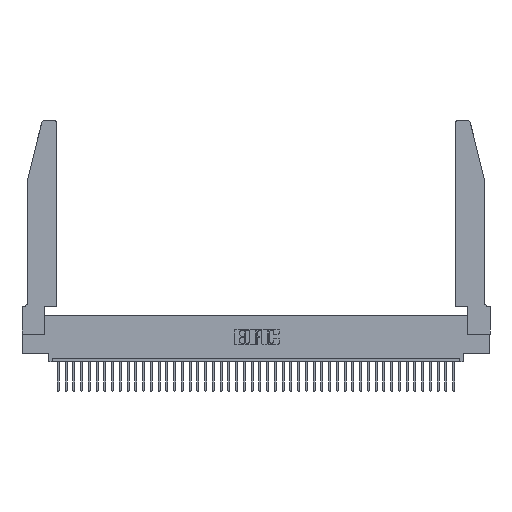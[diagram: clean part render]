
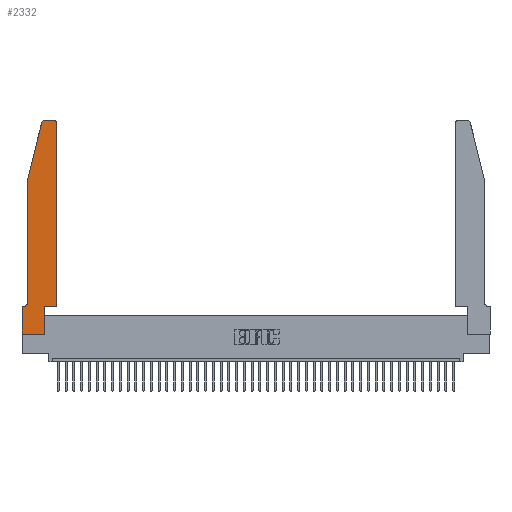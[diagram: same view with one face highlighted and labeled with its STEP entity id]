
A CAD part, top view. The second image highlights one B-rep face of the part: STEP entity #2332.
In plain terms, the highlighted planar face has unit normal (0, 0, 1).
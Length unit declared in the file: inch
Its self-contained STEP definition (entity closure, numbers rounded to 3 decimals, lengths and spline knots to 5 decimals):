
#23 = PLANE ( 'NONE',  #446 ) ;
#157 = DIRECTION ( 'NONE',  ( 1., 0., 0. ) ) ;
#178 = LINE ( 'NONE', #6188, #29043 ) ;
#213 = ORIENTED_EDGE ( 'NONE', *, *, #14156, .T. ) ;
#418 = ORIENTED_EDGE ( 'NONE', *, *, #34478, .T. ) ;
#446 = AXIS2_PLACEMENT_3D ( 'NONE', #26949, #29822, #157 ) ;
#1117 = CARTESIAN_POINT ( 'NONE',  ( 0., 0., 0.37 ) ) ;
#1742 = FACE_OUTER_BOUND ( 'NONE', #40626, .T. ) ;
#1917 = ORIENTED_EDGE ( 'NONE', *, *, #10054, .T. ) ;
#2095 = ORIENTED_EDGE ( 'NONE', *, *, #18398, .T. ) ;
#2332 = ADVANCED_FACE ( 'NONE', ( #1742 ), #23, .T. ) ;
#2423 = DIRECTION ( 'NONE',  ( 0., 1., 0. ) ) ;
#2573 = CARTESIAN_POINT ( 'NONE',  ( 0.2865, 0.35, 0.37 ) ) ;
#3105 = VERTEX_POINT ( 'NONE', #30296 ) ;
#3519 = AXIS2_PLACEMENT_3D ( 'NONE', #18840, #19130, #35691 ) ;
#4041 = EDGE_CURVE ( 'NONE', #3105, #24689, #11425, .T. ) ;
#4183 = CARTESIAN_POINT ( 'NONE',  ( 0.4505, 0.35, 0.37 ) ) ;
#4544 = CARTESIAN_POINT ( 'NONE',  ( 0.4205, 2.72, 0.37 ) ) ;
#4831 = EDGE_CURVE ( 'NONE', #13721, #42676, #30456, .T. ) ;
#4833 = DIRECTION ( 'NONE',  ( 0., 0., 1. ) ) ;
#5234 = CARTESIAN_POINT ( 'NONE',  ( 0.4205, 2.75, 0.37 ) ) ;
#5642 = EDGE_CURVE ( 'NONE', #30776, #18917, #25253, .T. ) ;
#6029 = LINE ( 'NONE', #32280, #40094 ) ;
#6188 = CARTESIAN_POINT ( 'NONE',  ( 0.4505, 0.35, 0.37 ) ) ;
#6521 = DIRECTION ( 'NONE',  ( -1., 0., 0. ) ) ;
#6997 = LINE ( 'NONE', #38324, #8029 ) ;
#7687 = LINE ( 'NONE', #28953, #13379 ) ;
#7872 = CARTESIAN_POINT ( 'NONE',  ( 0.25487, 2.72718, 0.37 ) ) ;
#8029 = VECTOR ( 'NONE', #15065, 39.37008 ) ;
#8715 = LINE ( 'NONE', #2573, #23701 ) ;
#9476 = DIRECTION ( 'NONE',  ( -1., 0., 0. ) ) ;
#9899 = VERTEX_POINT ( 'NONE', #38356 ) ;
#10054 = EDGE_CURVE ( 'NONE', #42676, #26106, #7687, .T. ) ;
#11241 = VECTOR ( 'NONE', #37070, 39.37008 ) ;
#11425 = LINE ( 'NONE', #27756, #39852 ) ;
#11808 = VERTEX_POINT ( 'NONE', #39655 ) ;
#12030 = EDGE_CURVE ( 'NONE', #26106, #30776, #6997, .T. ) ;
#12804 = ORIENTED_EDGE ( 'NONE', *, *, #19382, .T. ) ;
#13379 = VECTOR ( 'NONE', #22488, 39.37008 ) ;
#13721 = VERTEX_POINT ( 'NONE', #31810 ) ;
#14156 = EDGE_CURVE ( 'NONE', #11808, #21584, #38530, .T. ) ;
#14802 = CARTESIAN_POINT ( 'NONE',  ( 0.0755, 0.42, 0.37 ) ) ;
#15065 = DIRECTION ( 'NONE',  ( 0., -1., 0. ) ) ;
#15406 = LINE ( 'NONE', #4183, #11241 ) ;
#16074 = CARTESIAN_POINT ( 'NONE',  ( 0.0055, 0.42, 0.37 ) ) ;
#17065 = ORIENTED_EDGE ( 'NONE', *, *, #4041, .T. ) ;
#18398 = EDGE_CURVE ( 'NONE', #20252, #20653, #8715, .T. ) ;
#18840 = CARTESIAN_POINT ( 'NONE',  ( 0.284, 2.72, 0.37 ) ) ;
#18917 = VERTEX_POINT ( 'NONE', #34940 ) ;
#19130 = DIRECTION ( 'NONE',  ( 0., 0., 1. ) ) ;
#19382 = EDGE_CURVE ( 'NONE', #24689, #20252, #40137, .T. ) ;
#19650 = CARTESIAN_POINT ( 'NONE',  ( 0.2865, 0., 0.37 ) ) ;
#20036 = VECTOR ( 'NONE', #31714, 39.37008 ) ;
#20252 = VERTEX_POINT ( 'NONE', #19650 ) ;
#20653 = VERTEX_POINT ( 'NONE', #28682 ) ;
#20753 = ORIENTED_EDGE ( 'NONE', *, *, #4831, .T. ) ;
#21560 = ORIENTED_EDGE ( 'NONE', *, *, #27192, .T. ) ;
#21584 = VERTEX_POINT ( 'NONE', #5234 ) ;
#22488 = DIRECTION ( 'NONE',  ( -0.239, -0.971, 0. ) ) ;
#22776 = CARTESIAN_POINT ( 'NONE',  ( 0.2605, 2.75, 0.37 ) ) ;
#23701 = VECTOR ( 'NONE', #2423, 39.37008 ) ;
#24460 = EDGE_CURVE ( 'NONE', #20653, #9899, #178, .T. ) ;
#24689 = VERTEX_POINT ( 'NONE', #1117 ) ;
#25253 = CIRCLE ( 'NONE', #33739, 0.07 ) ;
#26106 = VERTEX_POINT ( 'NONE', #31081 ) ;
#26949 = CARTESIAN_POINT ( 'NONE',  ( 0., 0.35, 0.37 ) ) ;
#27192 = EDGE_CURVE ( 'NONE', #9899, #11808, #15406, .T. ) ;
#27292 = LINE ( 'NONE', #22776, #38676 ) ;
#27756 = CARTESIAN_POINT ( 'NONE',  ( 0., 0., 0.37 ) ) ;
#28682 = CARTESIAN_POINT ( 'NONE',  ( 0.2865, 0.35, 0.37 ) ) ;
#28953 = CARTESIAN_POINT ( 'NONE',  ( 0.0755, 2., 0.37 ) ) ;
#29043 = VECTOR ( 'NONE', #39250, 39.37008 ) ;
#29483 = DIRECTION ( 'NONE',  ( 0., 0., -1. ) ) ;
#29822 = DIRECTION ( 'NONE',  ( 0., 0., 1. ) ) ;
#30296 = CARTESIAN_POINT ( 'NONE',  ( 0., 0.35, 0.37 ) ) ;
#30313 = AXIS2_PLACEMENT_3D ( 'NONE', #4544, #4833, #31173 ) ;
#30456 = CIRCLE ( 'NONE', #3519, 0.03 ) ;
#30776 = VERTEX_POINT ( 'NONE', #14802 ) ;
#31048 = DIRECTION ( 'NONE',  ( 0., -1., 0. ) ) ;
#31081 = CARTESIAN_POINT ( 'NONE',  ( 0.0755, 2., 0.37 ) ) ;
#31173 = DIRECTION ( 'NONE',  ( 1., 0., 0. ) ) ;
#31714 = DIRECTION ( 'NONE',  ( 1., 0., 0. ) ) ;
#31810 = CARTESIAN_POINT ( 'NONE',  ( 0.284, 2.75, 0.37 ) ) ;
#32252 = ORIENTED_EDGE ( 'NONE', *, *, #12030, .T. ) ;
#32280 = CARTESIAN_POINT ( 'NONE',  ( 0.0755, 0.35, 0.37 ) ) ;
#33415 = EDGE_CURVE ( 'NONE', #21584, #13721, #27292, .T. ) ;
#33739 = AXIS2_PLACEMENT_3D ( 'NONE', #16074, #29483, #6521 ) ;
#34478 = EDGE_CURVE ( 'NONE', #18917, #3105, #6029, .T. ) ;
#34940 = CARTESIAN_POINT ( 'NONE',  ( 0.0055, 0.35, 0.37 ) ) ;
#35691 = DIRECTION ( 'NONE',  ( 1., 0., 0. ) ) ;
#37070 = DIRECTION ( 'NONE',  ( 0., 1., 0. ) ) ;
#37663 = ORIENTED_EDGE ( 'NONE', *, *, #24460, .T. ) ;
#38324 = CARTESIAN_POINT ( 'NONE',  ( 0.0755, 2., 0.37 ) ) ;
#38356 = CARTESIAN_POINT ( 'NONE',  ( 0.4505, 0.35, 0.37 ) ) ;
#38530 = CIRCLE ( 'NONE', #30313, 0.03 ) ;
#38676 = VECTOR ( 'NONE', #9476, 39.37008 ) ;
#38952 = DIRECTION ( 'NONE',  ( -1., 0., 0. ) ) ;
#39250 = DIRECTION ( 'NONE',  ( 1., 0., 0. ) ) ;
#39445 = ORIENTED_EDGE ( 'NONE', *, *, #5642, .T. ) ;
#39655 = CARTESIAN_POINT ( 'NONE',  ( 0.4505, 2.72, 0.37 ) ) ;
#39852 = VECTOR ( 'NONE', #31048, 39.37008 ) ;
#40094 = VECTOR ( 'NONE', #38952, 39.37008 ) ;
#40137 = LINE ( 'NONE', #41685, #20036 ) ;
#40626 = EDGE_LOOP ( 'NONE', ( #42238, #20753, #1917, #32252, #39445, #418, #17065, #12804, #2095, #37663, #21560, #213 ) ) ;
#41685 = CARTESIAN_POINT ( 'NONE',  ( 0., 0., 0.37 ) ) ;
#42238 = ORIENTED_EDGE ( 'NONE', *, *, #33415, .T. ) ;
#42676 = VERTEX_POINT ( 'NONE', #7872 ) ;
